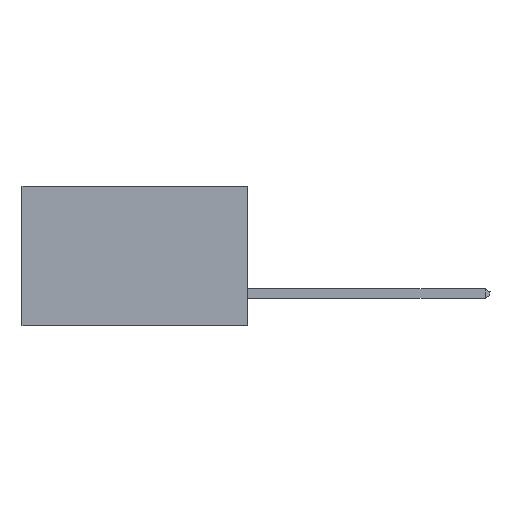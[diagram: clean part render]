
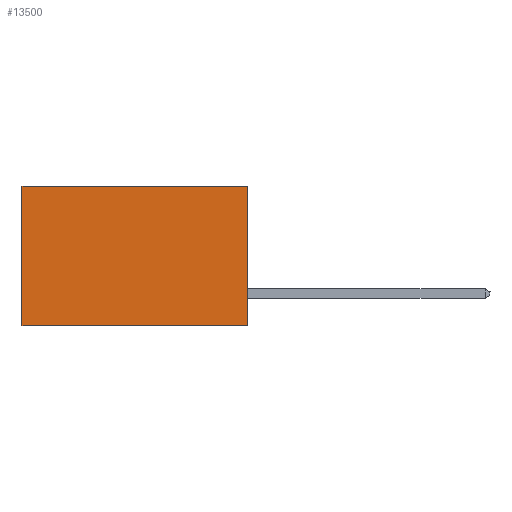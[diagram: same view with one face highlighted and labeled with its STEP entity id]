
A CAD part, left-side view. The second image highlights one B-rep face of the part: STEP entity #13500.
In plain terms, the highlighted planar face has unit normal (-1, 0, 0).
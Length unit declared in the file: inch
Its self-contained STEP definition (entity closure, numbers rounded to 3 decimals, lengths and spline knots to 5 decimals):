
#100 = LINE ( 'NONE', #16414, #8405 ) ;
#153 = EDGE_CURVE ( 'NONE', #965, #6058, #1996, .T. ) ;
#294 = ORIENTED_EDGE ( 'NONE', *, *, #16170, .F. ) ;
#886 = EDGE_LOOP ( 'NONE', ( #10830, #294, #19383, #1283 ) ) ;
#965 = VERTEX_POINT ( 'NONE', #8118 ) ;
#1126 = DIRECTION ( 'NONE',  ( 1., 0., 0. ) ) ;
#1283 = ORIENTED_EDGE ( 'NONE', *, *, #15330, .T. ) ;
#1996 = LINE ( 'NONE', #13709, #10256 ) ;
#2841 = DIRECTION ( 'NONE',  ( 0., 0., -1. ) ) ;
#3808 = DIRECTION ( 'NONE',  ( 0., 0., -1. ) ) ;
#4585 = AXIS2_PLACEMENT_3D ( 'NONE', #12659, #1126, #2841 ) ;
#5158 = VERTEX_POINT ( 'NONE', #6241 ) ;
#5164 = LINE ( 'NONE', #19885, #8708 ) ;
#5217 = DIRECTION ( 'NONE',  ( 0., 1., 0. ) ) ;
#5303 = LINE ( 'NONE', #18414, #11817 ) ;
#6058 = VERTEX_POINT ( 'NONE', #16214 ) ;
#6241 = CARTESIAN_POINT ( 'NONE',  ( 0.2615, 0.6, -0.37 ) ) ;
#8118 = CARTESIAN_POINT ( 'NONE',  ( 0.2615, 0., 0. ) ) ;
#8353 = DIRECTION ( 'NONE',  ( 0., 1., 0. ) ) ;
#8405 = VECTOR ( 'NONE', #5217, 39.37008 ) ;
#8708 = VECTOR ( 'NONE', #8353, 39.37008 ) ;
#10256 = VECTOR ( 'NONE', #11996, 39.37008 ) ;
#10830 = ORIENTED_EDGE ( 'NONE', *, *, #16815, .T. ) ;
#11817 = VECTOR ( 'NONE', #3808, 39.37008 ) ;
#11996 = DIRECTION ( 'NONE',  ( 0., 0., -1. ) ) ;
#12659 = CARTESIAN_POINT ( 'NONE',  ( 0.2615, 0., -0.37 ) ) ;
#13500 = ADVANCED_FACE ( 'NONE', ( #21092 ), #19492, .F. ) ;
#13709 = CARTESIAN_POINT ( 'NONE',  ( 0.2615, 0., -0.37 ) ) ;
#15193 = CARTESIAN_POINT ( 'NONE',  ( 0.2615, 0.6, 0. ) ) ;
#15330 = EDGE_CURVE ( 'NONE', #965, #15495, #5164, .T. ) ;
#15495 = VERTEX_POINT ( 'NONE', #15193 ) ;
#16170 = EDGE_CURVE ( 'NONE', #6058, #5158, #100, .T. ) ;
#16214 = CARTESIAN_POINT ( 'NONE',  ( 0.2615, 0., -0.37 ) ) ;
#16414 = CARTESIAN_POINT ( 'NONE',  ( 0.2615, 0., -0.37 ) ) ;
#16815 = EDGE_CURVE ( 'NONE', #15495, #5158, #5303, .T. ) ;
#18414 = CARTESIAN_POINT ( 'NONE',  ( 0.2615, 0.6, -0.37 ) ) ;
#19383 = ORIENTED_EDGE ( 'NONE', *, *, #153, .F. ) ;
#19492 = PLANE ( 'NONE',  #4585 ) ;
#19885 = CARTESIAN_POINT ( 'NONE',  ( 0.2615, 0., 0. ) ) ;
#21092 = FACE_OUTER_BOUND ( 'NONE', #886, .T. ) ;
